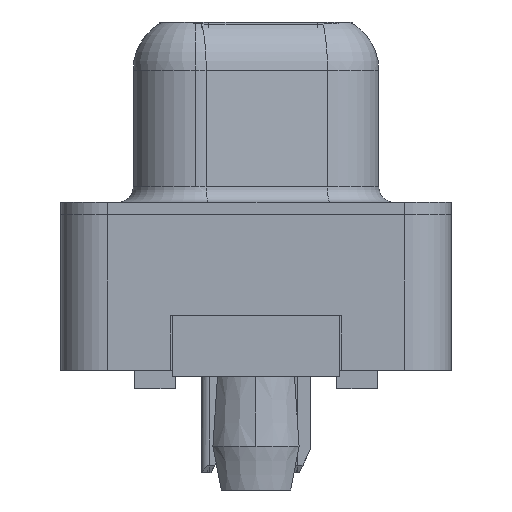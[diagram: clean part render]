
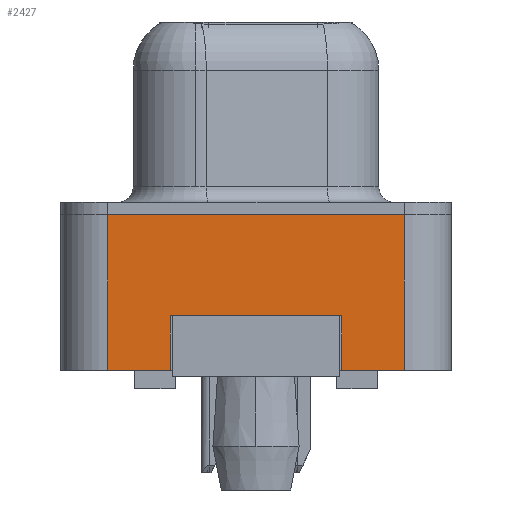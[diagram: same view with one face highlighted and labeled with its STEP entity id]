
A CAD part, left-side view. The second image highlights one B-rep face of the part: STEP entity #2427.
In plain terms, the highlighted planar face has unit normal (-1, 0, 0).
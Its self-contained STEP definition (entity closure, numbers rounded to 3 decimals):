
#135 = CARTESIAN_POINT ( 'NONE',  ( -2.945, -2.75, -3.25 ) ) ;
#598 = CARTESIAN_POINT ( 'NONE',  ( -2.945, -4.775, -5. ) ) ;
#930 = ORIENTED_EDGE ( 'NONE', *, *, #14292, .F. ) ;
#1152 = VERTEX_POINT ( 'NONE', #9127 ) ;
#1749 = EDGE_CURVE ( 'NONE', #8811, #13316, #8440, .T. ) ;
#2366 = CARTESIAN_POINT ( 'NONE',  ( -2.945, -4.775, -5. ) ) ;
#2426 = VECTOR ( 'NONE', #4346, 1000. ) ;
#2427 = ADVANCED_FACE ( 'NONE', ( #14665 ), #2724, .T. ) ;
#2571 = ORIENTED_EDGE ( 'NONE', *, *, #3792, .F. ) ;
#2724 = PLANE ( 'NONE',  #10995 ) ;
#2878 = VECTOR ( 'NONE', #9504, 1000. ) ;
#3792 = EDGE_CURVE ( 'NONE', #15627, #7188, #16737, .T. ) ;
#3991 = CARTESIAN_POINT ( 'NONE',  ( -2.945, 2.75, -3.25 ) ) ;
#4346 = DIRECTION ( 'NONE',  ( 0., -1., 0. ) ) ;
#4364 = CARTESIAN_POINT ( 'NONE',  ( -2.945, -2.75, -3.25 ) ) ;
#4576 = EDGE_CURVE ( 'NONE', #1152, #10815, #9728, .T. ) ;
#4722 = ORIENTED_EDGE ( 'NONE', *, *, #13921, .T. ) ;
#4802 = CARTESIAN_POINT ( 'NONE',  ( -2.945, -4.775, 0. ) ) ;
#5332 = DIRECTION ( 'NONE',  ( 0., 0., 1. ) ) ;
#5477 = VECTOR ( 'NONE', #5332, 1000. ) ;
#5651 = ORIENTED_EDGE ( 'NONE', *, *, #1749, .T. ) ;
#6059 = CARTESIAN_POINT ( 'NONE',  ( -2.945, -4.775, -5. ) ) ;
#6231 = VECTOR ( 'NONE', #7466, 1000. ) ;
#6609 = LINE ( 'NONE', #3991, #11753 ) ;
#6642 = EDGE_CURVE ( 'NONE', #8811, #12042, #16811, .T. ) ;
#7188 = VERTEX_POINT ( 'NONE', #13262 ) ;
#7466 = DIRECTION ( 'NONE',  ( 0., -1., 0. ) ) ;
#7908 = EDGE_CURVE ( 'NONE', #13316, #15908, #13584, .T. ) ;
#8440 = LINE ( 'NONE', #4364, #2878 ) ;
#8811 = VERTEX_POINT ( 'NONE', #135 ) ;
#8985 = CARTESIAN_POINT ( 'NONE',  ( -2.945, -4.775, -5. ) ) ;
#9127 = CARTESIAN_POINT ( 'NONE',  ( -2.945, 4.775, -5. ) ) ;
#9287 = DIRECTION ( 'NONE',  ( 0., 0., -1. ) ) ;
#9504 = DIRECTION ( 'NONE',  ( 0., 0., -1. ) ) ;
#9643 = CARTESIAN_POINT ( 'NONE',  ( -2.945, 2.75, -3.25 ) ) ;
#9728 = LINE ( 'NONE', #598, #6231 ) ;
#10113 = DIRECTION ( 'NONE',  ( 0., -1., 0. ) ) ;
#10161 = CARTESIAN_POINT ( 'NONE',  ( -2.945, -2.75, -5. ) ) ;
#10310 = DIRECTION ( 'NONE',  ( 0., 0., 1. ) ) ;
#10478 = CARTESIAN_POINT ( 'NONE',  ( -2.945, 4.775, 0. ) ) ;
#10772 = VECTOR ( 'NONE', #10113, 1000. ) ;
#10815 = VERTEX_POINT ( 'NONE', #16368 ) ;
#10995 = AXIS2_PLACEMENT_3D ( 'NONE', #8985, #14315, #10310 ) ;
#11107 = EDGE_CURVE ( 'NONE', #12042, #10815, #6609, .T. ) ;
#11375 = DIRECTION ( 'NONE',  ( 0., 0., 1. ) ) ;
#11753 = VECTOR ( 'NONE', #9287, 1000. ) ;
#11840 = DIRECTION ( 'NONE',  ( 0., 1., 0. ) ) ;
#12017 = CARTESIAN_POINT ( 'NONE',  ( -2.945, 2.75, -3.25 ) ) ;
#12042 = VERTEX_POINT ( 'NONE', #9643 ) ;
#12127 = CARTESIAN_POINT ( 'NONE',  ( -2.945, -4.775, -5. ) ) ;
#12425 = ORIENTED_EDGE ( 'NONE', *, *, #4576, .T. ) ;
#12679 = LINE ( 'NONE', #6059, #15754 ) ;
#12825 = ORIENTED_EDGE ( 'NONE', *, *, #11107, .F. ) ;
#13041 = EDGE_LOOP ( 'NONE', ( #5651, #14368, #4722, #2571, #930, #12425, #12825, #13454 ) ) ;
#13262 = CARTESIAN_POINT ( 'NONE',  ( -2.945, -4.775, 0. ) ) ;
#13316 = VERTEX_POINT ( 'NONE', #10161 ) ;
#13454 = ORIENTED_EDGE ( 'NONE', *, *, #6642, .F. ) ;
#13496 = VECTOR ( 'NONE', #11840, 1000. ) ;
#13584 = LINE ( 'NONE', #12127, #2426 ) ;
#13921 = EDGE_CURVE ( 'NONE', #15908, #7188, #12679, .T. ) ;
#14292 = EDGE_CURVE ( 'NONE', #1152, #15627, #14904, .T. ) ;
#14315 = DIRECTION ( 'NONE',  ( -1., 0., 0. ) ) ;
#14368 = ORIENTED_EDGE ( 'NONE', *, *, #7908, .T. ) ;
#14657 = CARTESIAN_POINT ( 'NONE',  ( -2.945, 4.775, -5. ) ) ;
#14665 = FACE_OUTER_BOUND ( 'NONE', #13041, .T. ) ;
#14904 = LINE ( 'NONE', #14657, #5477 ) ;
#15627 = VERTEX_POINT ( 'NONE', #10478 ) ;
#15754 = VECTOR ( 'NONE', #11375, 1000. ) ;
#15908 = VERTEX_POINT ( 'NONE', #2366 ) ;
#16368 = CARTESIAN_POINT ( 'NONE',  ( -2.945, 2.75, -5. ) ) ;
#16737 = LINE ( 'NONE', #4802, #10772 ) ;
#16811 = LINE ( 'NONE', #12017, #13496 ) ;
